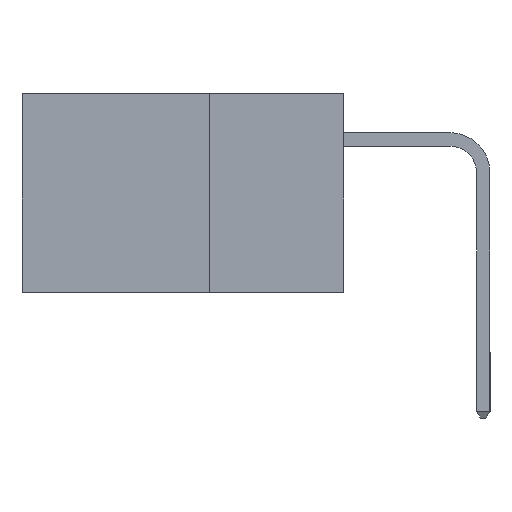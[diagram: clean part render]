
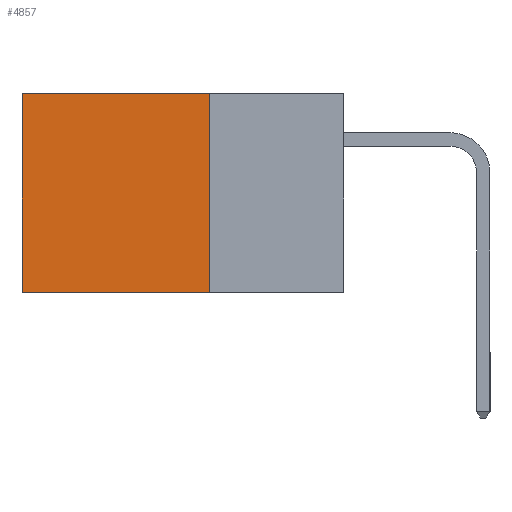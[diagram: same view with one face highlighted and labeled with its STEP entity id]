
A CAD part, left-side view. The second image highlights one B-rep face of the part: STEP entity #4857.
In plain terms, the highlighted planar face has unit normal (-1, 0, 0).
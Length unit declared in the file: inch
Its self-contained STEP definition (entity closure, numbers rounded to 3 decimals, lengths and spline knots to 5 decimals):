
#1311 = LINE ( 'NONE', #15000, #24116 ) ;
#3542 = ORIENTED_EDGE ( 'NONE', *, *, #22441, .T. ) ;
#4299 = LINE ( 'NONE', #17897, #30843 ) ;
#4423 = VERTEX_POINT ( 'NONE', #11882 ) ;
#4491 = DIRECTION ( 'NONE',  ( 0., 0., -1. ) ) ;
#4653 = AXIS2_PLACEMENT_3D ( 'NONE', #28614, #23776, #13857 ) ;
#4857 = ADVANCED_FACE ( 'NONE', ( #12924 ), #26123, .F. ) ;
#6296 = CARTESIAN_POINT ( 'NONE',  ( 0.298, 0.6, 0. ) ) ;
#8072 = CARTESIAN_POINT ( 'NONE',  ( 0.298, 0.25, 0. ) ) ;
#8309 = VERTEX_POINT ( 'NONE', #6296 ) ;
#9181 = DIRECTION ( 'NONE',  ( 0., 0., -1. ) ) ;
#9404 = CARTESIAN_POINT ( 'NONE',  ( 0.298, 0.6, 0. ) ) ;
#9684 = CARTESIAN_POINT ( 'NONE',  ( 0.298, 0.6, -0.37 ) ) ;
#9941 = ORIENTED_EDGE ( 'NONE', *, *, #27421, .F. ) ;
#10262 = ORIENTED_EDGE ( 'NONE', *, *, #23169, .F. ) ;
#11882 = CARTESIAN_POINT ( 'NONE',  ( 0.298, 0.25, -0.37 ) ) ;
#12271 = EDGE_LOOP ( 'NONE', ( #3542, #10262, #9941, #18197 ) ) ;
#12924 = FACE_OUTER_BOUND ( 'NONE', #12271, .T. ) ;
#13857 = DIRECTION ( 'NONE',  ( 0., 0., -1. ) ) ;
#15000 = CARTESIAN_POINT ( 'NONE',  ( 0.298, 0.25, -0.37 ) ) ;
#17897 = CARTESIAN_POINT ( 'NONE',  ( 0.298, 0.25, 0. ) ) ;
#18197 = ORIENTED_EDGE ( 'NONE', *, *, #19547, .T. ) ;
#19540 = DIRECTION ( 'NONE',  ( 0., 1., 0. ) ) ;
#19547 = EDGE_CURVE ( 'NONE', #30397, #8309, #4299, .T. ) ;
#20277 = DIRECTION ( 'NONE',  ( 0., 1., 0. ) ) ;
#22441 = EDGE_CURVE ( 'NONE', #8309, #29534, #26854, .T. ) ;
#23169 = EDGE_CURVE ( 'NONE', #4423, #29534, #1311, .T. ) ;
#23776 = DIRECTION ( 'NONE',  ( 1., 0., 0. ) ) ;
#24083 = CARTESIAN_POINT ( 'NONE',  ( 0.298, 0.25, 0. ) ) ;
#24116 = VECTOR ( 'NONE', #19540, 39.37008 ) ;
#24550 = VECTOR ( 'NONE', #9181, 39.37008 ) ;
#25538 = VECTOR ( 'NONE', #4491, 39.37008 ) ;
#26123 = PLANE ( 'NONE',  #4653 ) ;
#26854 = LINE ( 'NONE', #9404, #24550 ) ;
#27421 = EDGE_CURVE ( 'NONE', #30397, #4423, #29021, .T. ) ;
#28614 = CARTESIAN_POINT ( 'NONE',  ( 0.298, 0.25, 0. ) ) ;
#29021 = LINE ( 'NONE', #24083, #25538 ) ;
#29534 = VERTEX_POINT ( 'NONE', #9684 ) ;
#30397 = VERTEX_POINT ( 'NONE', #8072 ) ;
#30843 = VECTOR ( 'NONE', #20277, 39.37008 ) ;
